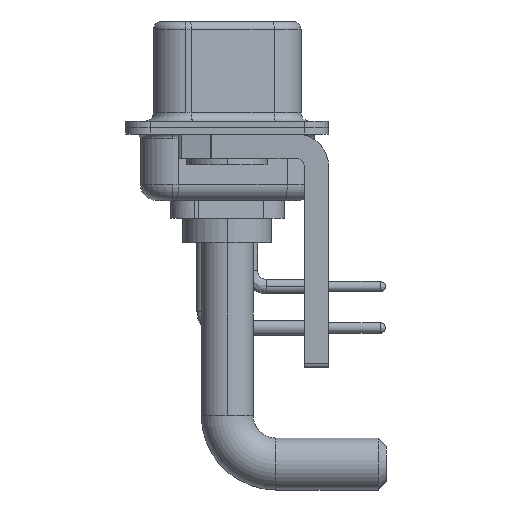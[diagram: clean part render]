
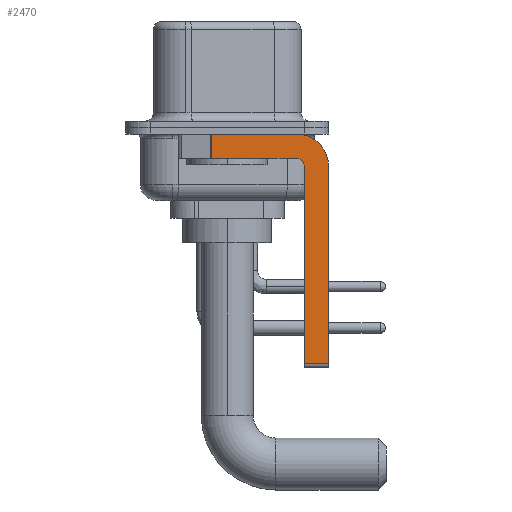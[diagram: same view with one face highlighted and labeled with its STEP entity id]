
A CAD part, left-side view. The second image highlights one B-rep face of the part: STEP entity #2470.
In plain terms, the highlighted planar face has unit normal (-1, 0, 0).
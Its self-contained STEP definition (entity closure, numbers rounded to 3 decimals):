
#199 = EDGE_CURVE ( 'NONE', #7219, #13582, #3304, .T. ) ;
#1002 = AXIS2_PLACEMENT_3D ( 'NONE', #24300, #1805, #4259 ) ;
#1644 = AXIS2_PLACEMENT_3D ( 'NONE', #20386, #16167, #11390 ) ;
#1710 = VERTEX_POINT ( 'NONE', #2203 ) ;
#1805 = DIRECTION ( 'NONE',  ( 1., 0., 0. ) ) ;
#1835 = CARTESIAN_POINT ( 'NONE',  ( -2.9, 0.978, -1.9 ) ) ;
#2203 = CARTESIAN_POINT ( 'NONE',  ( -2.9, -6.25, -14.55 ) ) ;
#2470 = ADVANCED_FACE ( 'NONE', ( #17354 ), #17195, .F. ) ;
#3304 = LINE ( 'NONE', #23048, #24128 ) ;
#4047 = EDGE_CURVE ( 'NONE', #13377, #21855, #9429, .T. ) ;
#4259 = DIRECTION ( 'NONE',  ( 0., 0., -1. ) ) ;
#4790 = CARTESIAN_POINT ( 'NONE',  ( -2.9, 3., -0.4 ) ) ;
#5055 = DIRECTION ( 'NONE',  ( 0., -1., 0. ) ) ;
#5163 = CIRCLE ( 'NONE', #21397, 2. ) ;
#6652 = LINE ( 'NONE', #15516, #10591 ) ;
#6912 = VECTOR ( 'NONE', #27352, 1000. ) ;
#7219 = VERTEX_POINT ( 'NONE', #11102 ) ;
#7418 = VECTOR ( 'NONE', #19011, 1000. ) ;
#7852 = ORIENTED_EDGE ( 'NONE', *, *, #13882, .F. ) ;
#7960 = EDGE_LOOP ( 'NONE', ( #25709, #27304, #15600, #17602, #8821, #24189, #7852, #26493 ) ) ;
#8281 = DIRECTION ( 'NONE',  ( 0., 0., -1. ) ) ;
#8821 = ORIENTED_EDGE ( 'NONE', *, *, #19682, .F. ) ;
#9113 = CARTESIAN_POINT ( 'NONE',  ( -2.9, -4.75, -2.4 ) ) ;
#9429 = LINE ( 'NONE', #4790, #13602 ) ;
#10442 = CARTESIAN_POINT ( 'NONE',  ( -2.9, -4.25, -14.55 ) ) ;
#10591 = VECTOR ( 'NONE', #20019, 1000. ) ;
#11102 = CARTESIAN_POINT ( 'NONE',  ( -2.9, -4.25, -1.9 ) ) ;
#11390 = DIRECTION ( 'NONE',  ( 0., 0., 1. ) ) ;
#12219 = CARTESIAN_POINT ( 'NONE',  ( -2.9, 0.978, -1.9 ) ) ;
#12389 = EDGE_CURVE ( 'NONE', #28412, #7219, #27142, .T. ) ;
#12394 = CARTESIAN_POINT ( 'NONE',  ( -2.9, -4.75, -14.55 ) ) ;
#13377 = VERTEX_POINT ( 'NONE', #24794 ) ;
#13582 = VERTEX_POINT ( 'NONE', #1835 ) ;
#13602 = VECTOR ( 'NONE', #5055, 1000. ) ;
#13865 = LINE ( 'NONE', #16193, #6912 ) ;
#13882 = EDGE_CURVE ( 'NONE', #21934, #1710, #13865, .T. ) ;
#15516 = CARTESIAN_POINT ( 'NONE',  ( -2.9, -4.75, -14.8 ) ) ;
#15600 = ORIENTED_EDGE ( 'NONE', *, *, #199, .F. ) ;
#16103 = EDGE_CURVE ( 'NONE', #21855, #21934, #5163, .T. ) ;
#16167 = DIRECTION ( 'NONE',  ( -1., 0., 0. ) ) ;
#16193 = CARTESIAN_POINT ( 'NONE',  ( -2.9, -6.25, -2.4 ) ) ;
#17195 = PLANE ( 'NONE',  #1002 ) ;
#17354 = FACE_OUTER_BOUND ( 'NONE', #7960, .T. ) ;
#17602 = ORIENTED_EDGE ( 'NONE', *, *, #12389, .F. ) ;
#18773 = CARTESIAN_POINT ( 'NONE',  ( -2.9, -4.25, -2.4 ) ) ;
#19011 = DIRECTION ( 'NONE',  ( 0., -1., 0. ) ) ;
#19682 = EDGE_CURVE ( 'NONE', #21498, #28412, #6652, .T. ) ;
#20019 = DIRECTION ( 'NONE',  ( 0., 0., 1. ) ) ;
#20386 = CARTESIAN_POINT ( 'NONE',  ( -2.9, -4.25, -2.4 ) ) ;
#21397 = AXIS2_PLACEMENT_3D ( 'NONE', #18773, #27616, #25423 ) ;
#21498 = VERTEX_POINT ( 'NONE', #12394 ) ;
#21855 = VERTEX_POINT ( 'NONE', #22239 ) ;
#21934 = VERTEX_POINT ( 'NONE', #24512 ) ;
#22239 = CARTESIAN_POINT ( 'NONE',  ( -2.9, -4.25, -0.4 ) ) ;
#23048 = CARTESIAN_POINT ( 'NONE',  ( -2.9, -4.25, -1.9 ) ) ;
#24128 = VECTOR ( 'NONE', #25243, 1000. ) ;
#24189 = ORIENTED_EDGE ( 'NONE', *, *, #24750, .T. ) ;
#24190 = VECTOR ( 'NONE', #8281, 1000. ) ;
#24269 = EDGE_CURVE ( 'NONE', #13377, #13582, #25844, .T. ) ;
#24300 = CARTESIAN_POINT ( 'NONE',  ( -2.9, -4.25, -2.4 ) ) ;
#24512 = CARTESIAN_POINT ( 'NONE',  ( -2.9, -6.25, -2.4 ) ) ;
#24750 = EDGE_CURVE ( 'NONE', #21498, #1710, #25950, .T. ) ;
#24794 = CARTESIAN_POINT ( 'NONE',  ( -2.9, 0.978, -0.4 ) ) ;
#25243 = DIRECTION ( 'NONE',  ( 0., 1., 0. ) ) ;
#25423 = DIRECTION ( 'NONE',  ( 0., 0., -1. ) ) ;
#25709 = ORIENTED_EDGE ( 'NONE', *, *, #4047, .F. ) ;
#25844 = LINE ( 'NONE', #12219, #24190 ) ;
#25950 = LINE ( 'NONE', #10442, #7418 ) ;
#26493 = ORIENTED_EDGE ( 'NONE', *, *, #16103, .F. ) ;
#27142 = CIRCLE ( 'NONE', #1644, 0.5 ) ;
#27304 = ORIENTED_EDGE ( 'NONE', *, *, #24269, .T. ) ;
#27352 = DIRECTION ( 'NONE',  ( 0., 0., -1. ) ) ;
#27616 = DIRECTION ( 'NONE',  ( 1., 0., 0. ) ) ;
#28412 = VERTEX_POINT ( 'NONE', #9113 ) ;
